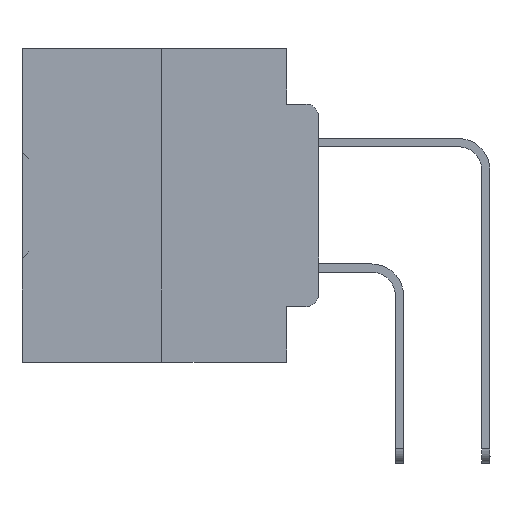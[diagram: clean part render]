
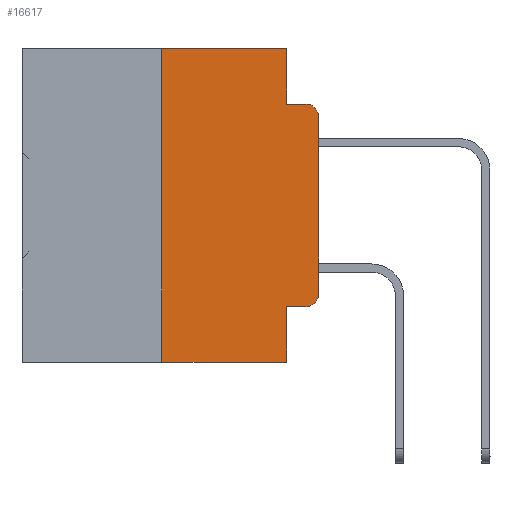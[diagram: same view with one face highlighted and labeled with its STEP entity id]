
A CAD part, left-side view. The second image highlights one B-rep face of the part: STEP entity #16617.
In plain terms, the highlighted planar face has unit normal (-1, 0, 0).
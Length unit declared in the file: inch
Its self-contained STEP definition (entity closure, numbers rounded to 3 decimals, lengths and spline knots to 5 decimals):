
#653 = EDGE_CURVE ( 'NONE', #33993, #33236, #5971, .T. ) ;
#939 = AXIS2_PLACEMENT_3D ( 'NONE', #35425, #31527, #16573 ) ;
#1366 = AXIS2_PLACEMENT_3D ( 'NONE', #30139, #3197, #6358 ) ;
#1724 = CARTESIAN_POINT ( 'NONE',  ( 0., 0.02, -0.0885 ) ) ;
#2623 = CARTESIAN_POINT ( 'NONE',  ( 0., 0.473, -0.5 ) ) ;
#3197 = DIRECTION ( 'NONE',  ( 1., 0., 0. ) ) ;
#4449 = VECTOR ( 'NONE', #12142, 39.37008 ) ;
#4666 = EDGE_CURVE ( 'NONE', #26976, #10257, #34980, .T. ) ;
#4927 = ORIENTED_EDGE ( 'NONE', *, *, #38721, .T. ) ;
#5120 = VERTEX_POINT ( 'NONE', #1724 ) ;
#5156 = CARTESIAN_POINT ( 'NONE',  ( 0., 0.02, -0.4115 ) ) ;
#5971 = CIRCLE ( 'NONE', #939, 0.02 ) ;
#6063 = CARTESIAN_POINT ( 'NONE',  ( 0., 0.051, -0.4115 ) ) ;
#6358 = DIRECTION ( 'NONE',  ( 0., 0., -1. ) ) ;
#6415 = VECTOR ( 'NONE', #34397, 39.37008 ) ;
#6817 = CARTESIAN_POINT ( 'NONE',  ( 0., 0., 0. ) ) ;
#6882 = EDGE_CURVE ( 'NONE', #33236, #33545, #9564, .T. ) ;
#7433 = ORIENTED_EDGE ( 'NONE', *, *, #37946, .F. ) ;
#7916 = VECTOR ( 'NONE', #29727, 39.37008 ) ;
#8195 = CARTESIAN_POINT ( 'NONE',  ( 0., 0.051, 0. ) ) ;
#8237 = AXIS2_PLACEMENT_3D ( 'NONE', #33879, #36234, #12253 ) ;
#8592 = ORIENTED_EDGE ( 'NONE', *, *, #653, .T. ) ;
#8784 = LINE ( 'NONE', #15056, #18123 ) ;
#8799 = VECTOR ( 'NONE', #18956, 39.37008 ) ;
#8954 = LINE ( 'NONE', #36053, #8799 ) ;
#8971 = EDGE_CURVE ( 'NONE', #35642, #28240, #32674, .T. ) ;
#9564 = LINE ( 'NONE', #6817, #15398 ) ;
#9837 = CARTESIAN_POINT ( 'NONE',  ( 0., 0.25, -0.5 ) ) ;
#9851 = DIRECTION ( 'NONE',  ( 0., -1., 0. ) ) ;
#10257 = VERTEX_POINT ( 'NONE', #19342 ) ;
#11651 = CARTESIAN_POINT ( 'NONE',  ( 0., 0.051, 0. ) ) ;
#11806 = EDGE_CURVE ( 'NONE', #29185, #12715, #8784, .T. ) ;
#12142 = DIRECTION ( 'NONE',  ( 0., -1., 0. ) ) ;
#12149 = CARTESIAN_POINT ( 'NONE',  ( 0., 0.051, -0.5 ) ) ;
#12253 = DIRECTION ( 'NONE',  ( 0., 0., -1. ) ) ;
#12715 = VERTEX_POINT ( 'NONE', #37188 ) ;
#13784 = EDGE_CURVE ( 'NONE', #33545, #5120, #37089, .T. ) ;
#15056 = CARTESIAN_POINT ( 'NONE',  ( 0., 0.25, 0. ) ) ;
#15398 = VECTOR ( 'NONE', #24514, 39.37008 ) ;
#15472 = LINE ( 'NONE', #6063, #4449 ) ;
#15847 = ORIENTED_EDGE ( 'NONE', *, *, #11806, .F. ) ;
#16573 = DIRECTION ( 'NONE',  ( 0., 0., -1. ) ) ;
#16617 = ADVANCED_FACE ( 'NONE', ( #24049 ), #36010, .F. ) ;
#17556 = LINE ( 'NONE', #2623, #35023 ) ;
#17646 = VECTOR ( 'NONE', #9851, 39.37008 ) ;
#18123 = VECTOR ( 'NONE', #26276, 39.37008 ) ;
#18956 = DIRECTION ( 'NONE',  ( 0., -1., 0. ) ) ;
#19342 = CARTESIAN_POINT ( 'NONE',  ( 0., 0.051, -0.0885 ) ) ;
#20169 = EDGE_CURVE ( 'NONE', #12715, #26976, #31071, .T. ) ;
#20994 = ORIENTED_EDGE ( 'NONE', *, *, #4666, .F. ) ;
#21319 = ORIENTED_EDGE ( 'NONE', *, *, #6882, .T. ) ;
#22216 = CARTESIAN_POINT ( 'NONE',  ( 0., 0.051, 0. ) ) ;
#23290 = CARTESIAN_POINT ( 'NONE',  ( 0., 0., -0.1085 ) ) ;
#24049 = FACE_OUTER_BOUND ( 'NONE', #25008, .T. ) ;
#24514 = DIRECTION ( 'NONE',  ( 0., 0., 1. ) ) ;
#25008 = EDGE_LOOP ( 'NONE', ( #21319, #33385, #7433, #20994, #32144, #15847, #34033, #37432, #4927, #8592 ) ) ;
#26276 = DIRECTION ( 'NONE',  ( 0., 0., 1. ) ) ;
#26976 = VERTEX_POINT ( 'NONE', #8195 ) ;
#28240 = VERTEX_POINT ( 'NONE', #12149 ) ;
#28931 = EDGE_CURVE ( 'NONE', #29185, #28240, #17556, .T. ) ;
#29185 = VERTEX_POINT ( 'NONE', #9837 ) ;
#29727 = DIRECTION ( 'NONE',  ( 0., 0., -1. ) ) ;
#30139 = CARTESIAN_POINT ( 'NONE',  ( 0., 0.473, 0. ) ) ;
#30874 = CARTESIAN_POINT ( 'NONE',  ( 0., 0.051, -0.4115 ) ) ;
#31071 = LINE ( 'NONE', #36768, #17646 ) ;
#31527 = DIRECTION ( 'NONE',  ( -1., 0., 0. ) ) ;
#32144 = ORIENTED_EDGE ( 'NONE', *, *, #20169, .F. ) ;
#32674 = LINE ( 'NONE', #11651, #7916 ) ;
#33141 = CARTESIAN_POINT ( 'NONE',  ( 0., 0., -0.3915 ) ) ;
#33236 = VERTEX_POINT ( 'NONE', #33141 ) ;
#33385 = ORIENTED_EDGE ( 'NONE', *, *, #13784, .T. ) ;
#33545 = VERTEX_POINT ( 'NONE', #23290 ) ;
#33879 = CARTESIAN_POINT ( 'NONE',  ( 0., 0.02, -0.1085 ) ) ;
#33993 = VERTEX_POINT ( 'NONE', #5156 ) ;
#34033 = ORIENTED_EDGE ( 'NONE', *, *, #28931, .T. ) ;
#34397 = DIRECTION ( 'NONE',  ( 0., 0., -1. ) ) ;
#34864 = DIRECTION ( 'NONE',  ( 0., -1., 0. ) ) ;
#34980 = LINE ( 'NONE', #22216, #6415 ) ;
#35023 = VECTOR ( 'NONE', #34864, 39.37008 ) ;
#35425 = CARTESIAN_POINT ( 'NONE',  ( 0., 0.02, -0.3915 ) ) ;
#35642 = VERTEX_POINT ( 'NONE', #30874 ) ;
#36010 = PLANE ( 'NONE',  #1366 ) ;
#36053 = CARTESIAN_POINT ( 'NONE',  ( 0., 0.051, -0.0885 ) ) ;
#36234 = DIRECTION ( 'NONE',  ( -1., 0., 0. ) ) ;
#36768 = CARTESIAN_POINT ( 'NONE',  ( 0., 0.473, 0. ) ) ;
#37089 = CIRCLE ( 'NONE', #8237, 0.02 ) ;
#37188 = CARTESIAN_POINT ( 'NONE',  ( 0., 0.25, 0. ) ) ;
#37432 = ORIENTED_EDGE ( 'NONE', *, *, #8971, .F. ) ;
#37946 = EDGE_CURVE ( 'NONE', #10257, #5120, #8954, .T. ) ;
#38721 = EDGE_CURVE ( 'NONE', #35642, #33993, #15472, .T. ) ;
